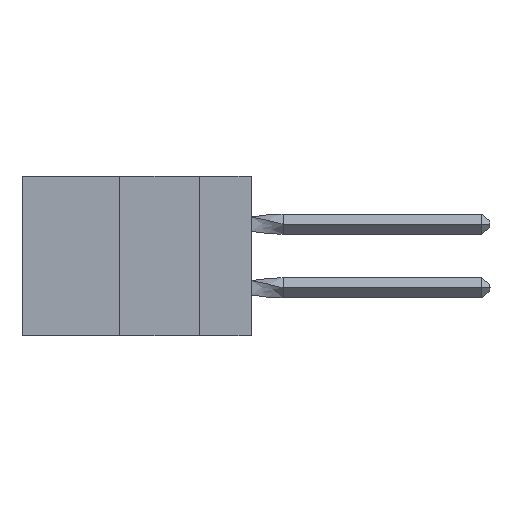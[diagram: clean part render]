
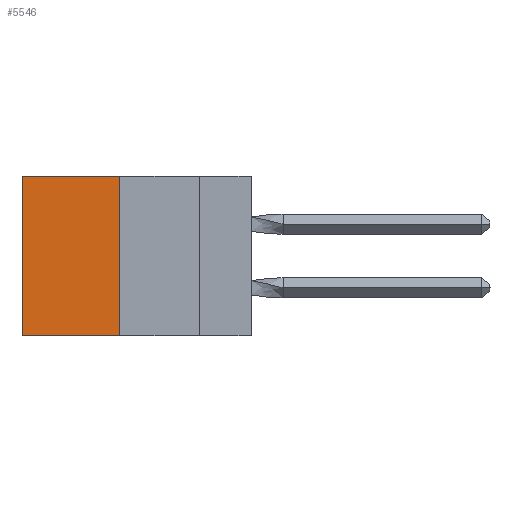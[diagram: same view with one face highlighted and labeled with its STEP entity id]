
A CAD part, left-side view. The second image highlights one B-rep face of the part: STEP entity #5546.
In plain terms, the highlighted planar face has unit normal (-1, 0, 0).
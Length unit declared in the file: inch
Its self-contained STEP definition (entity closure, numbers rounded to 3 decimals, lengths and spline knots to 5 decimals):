
#674 = CARTESIAN_POINT ( 'NONE',  ( 0.305, 0.413, 0. ) ) ;
#2116 = LINE ( 'NONE', #2373, #9259 ) ;
#2373 = CARTESIAN_POINT ( 'NONE',  ( 0.305, 0.413, -0.5 ) ) ;
#2444 = EDGE_CURVE ( 'NONE', #14891, #23691, #16629, .T. ) ;
#3366 = DIRECTION ( 'NONE',  ( 1., 0., 0. ) ) ;
#4824 = EDGE_CURVE ( 'NONE', #31774, #23691, #2116, .T. ) ;
#5546 = ADVANCED_FACE ( 'NONE', ( #31810 ), #18381, .F. ) ;
#5779 = LINE ( 'NONE', #15498, #14339 ) ;
#6024 = ORIENTED_EDGE ( 'NONE', *, *, #39165, .F. ) ;
#8254 = CARTESIAN_POINT ( 'NONE',  ( 0.305, 0.72, -0.5 ) ) ;
#9259 = VECTOR ( 'NONE', #39433, 39.37008 ) ;
#11261 = LINE ( 'NONE', #12947, #14573 ) ;
#12418 = ORIENTED_EDGE ( 'NONE', *, *, #2444, .T. ) ;
#12734 = CARTESIAN_POINT ( 'NONE',  ( 0.305, 0.72, 0. ) ) ;
#12947 = CARTESIAN_POINT ( 'NONE',  ( 0.305, 0.413, 0. ) ) ;
#13544 = EDGE_LOOP ( 'NONE', ( #12418, #31853, #6024, #22781 ) ) ;
#14339 = VECTOR ( 'NONE', #28156, 39.37008 ) ;
#14573 = VECTOR ( 'NONE', #16578, 39.37008 ) ;
#14891 = VERTEX_POINT ( 'NONE', #12734 ) ;
#15498 = CARTESIAN_POINT ( 'NONE',  ( 0.305, 0.413, -0.5 ) ) ;
#16209 = CARTESIAN_POINT ( 'NONE',  ( 0.305, 0.413, -0.5 ) ) ;
#16578 = DIRECTION ( 'NONE',  ( 0., 1., 0. ) ) ;
#16629 = LINE ( 'NONE', #38187, #39764 ) ;
#18381 = PLANE ( 'NONE',  #32327 ) ;
#22781 = ORIENTED_EDGE ( 'NONE', *, *, #34212, .T. ) ;
#23691 = VERTEX_POINT ( 'NONE', #8254 ) ;
#24199 = DIRECTION ( 'NONE',  ( 0., 0., -1. ) ) ;
#28156 = DIRECTION ( 'NONE',  ( 0., 0., -1. ) ) ;
#31774 = VERTEX_POINT ( 'NONE', #16209 ) ;
#31810 = FACE_OUTER_BOUND ( 'NONE', #13544, .T. ) ;
#31853 = ORIENTED_EDGE ( 'NONE', *, *, #4824, .F. ) ;
#32327 = AXIS2_PLACEMENT_3D ( 'NONE', #34003, #3366, #33852 ) ;
#33852 = DIRECTION ( 'NONE',  ( 0., 0., -1. ) ) ;
#34003 = CARTESIAN_POINT ( 'NONE',  ( 0.305, 0.413, -0.5 ) ) ;
#34212 = EDGE_CURVE ( 'NONE', #39106, #14891, #11261, .T. ) ;
#38187 = CARTESIAN_POINT ( 'NONE',  ( 0.305, 0.72, -0.5 ) ) ;
#39106 = VERTEX_POINT ( 'NONE', #674 ) ;
#39165 = EDGE_CURVE ( 'NONE', #39106, #31774, #5779, .T. ) ;
#39433 = DIRECTION ( 'NONE',  ( 0., 1., 0. ) ) ;
#39764 = VECTOR ( 'NONE', #24199, 39.37008 ) ;
